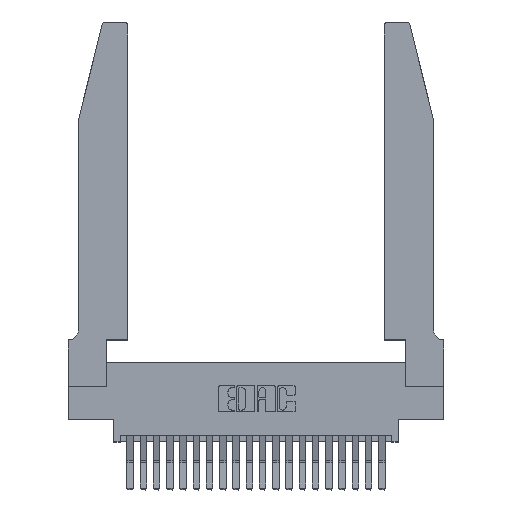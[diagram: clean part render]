
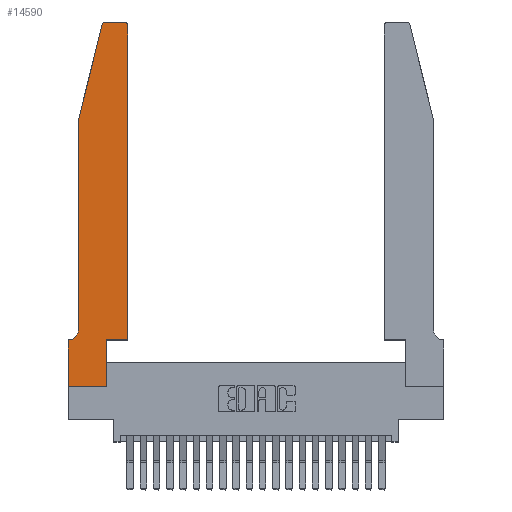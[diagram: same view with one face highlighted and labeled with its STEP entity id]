
A CAD part, top view. The second image highlights one B-rep face of the part: STEP entity #14590.
In plain terms, the highlighted planar face has unit normal (0, 0, 1).
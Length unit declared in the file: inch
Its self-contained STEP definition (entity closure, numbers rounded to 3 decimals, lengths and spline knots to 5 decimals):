
#285 = CARTESIAN_POINT ( 'NONE',  ( 0.4505, 0.35, 0.37 ) ) ;
#601 = VERTEX_POINT ( 'NONE', #14950 ) ;
#890 = LINE ( 'NONE', #285, #14241 ) ;
#1295 = LINE ( 'NONE', #7377, #20092 ) ;
#1777 = CIRCLE ( 'NONE', #19327, 0.03 ) ;
#1810 = VERTEX_POINT ( 'NONE', #23655 ) ;
#1978 = CARTESIAN_POINT ( 'NONE',  ( 0.284, 2.72, 0.37 ) ) ;
#2127 = AXIS2_PLACEMENT_3D ( 'NONE', #1978, #16276, #14726 ) ;
#3044 = LINE ( 'NONE', #10957, #20736 ) ;
#3111 = CARTESIAN_POINT ( 'NONE',  ( 0.0055, 0.35, 0.37 ) ) ;
#3375 = EDGE_CURVE ( 'NONE', #19369, #8964, #22174, .T. ) ;
#3530 = CARTESIAN_POINT ( 'NONE',  ( 0.0755, 2., 0.37 ) ) ;
#3537 = LINE ( 'NONE', #9108, #23262 ) ;
#3721 = LINE ( 'NONE', #5532, #21436 ) ;
#4109 = EDGE_CURVE ( 'NONE', #8964, #20138, #1295, .T. ) ;
#4708 = VECTOR ( 'NONE', #10912, 39.37008 ) ;
#5532 = CARTESIAN_POINT ( 'NONE',  ( 0.0755, 2., 0.37 ) ) ;
#5717 = EDGE_CURVE ( 'NONE', #11698, #6690, #1777, .T. ) ;
#5943 = CARTESIAN_POINT ( 'NONE',  ( 0.2865, 0., 0.37 ) ) ;
#6015 = VERTEX_POINT ( 'NONE', #3111 ) ;
#6218 = DIRECTION ( 'NONE',  ( 0., 0., -1. ) ) ;
#6465 = CARTESIAN_POINT ( 'NONE',  ( 0., 0., 0.37 ) ) ;
#6519 = DIRECTION ( 'NONE',  ( 0., 0., 1. ) ) ;
#6690 = VERTEX_POINT ( 'NONE', #17629 ) ;
#6797 = CARTESIAN_POINT ( 'NONE',  ( 0., 0.35, 0.37 ) ) ;
#6894 = DIRECTION ( 'NONE',  ( 1., 0., 0. ) ) ;
#7010 = VECTOR ( 'NONE', #17086, 39.37008 ) ;
#7377 = CARTESIAN_POINT ( 'NONE',  ( 0., 0., 0.37 ) ) ;
#7633 = ORIENTED_EDGE ( 'NONE', *, *, #7678, .T. ) ;
#7678 = EDGE_CURVE ( 'NONE', #6015, #19369, #12638, .T. ) ;
#7726 = ORIENTED_EDGE ( 'NONE', *, *, #22436, .T. ) ;
#7731 = DIRECTION ( 'NONE',  ( -1., 0., 0. ) ) ;
#8350 = CARTESIAN_POINT ( 'NONE',  ( 0.284, 2.75, 0.37 ) ) ;
#8524 = CARTESIAN_POINT ( 'NONE',  ( 0., 0.35, 0.37 ) ) ;
#8791 = ORIENTED_EDGE ( 'NONE', *, *, #10502, .T. ) ;
#8905 = EDGE_CURVE ( 'NONE', #19988, #6015, #12291, .T. ) ;
#8915 = ORIENTED_EDGE ( 'NONE', *, *, #17233, .T. ) ;
#8924 = ORIENTED_EDGE ( 'NONE', *, *, #3375, .T. ) ;
#8964 = VERTEX_POINT ( 'NONE', #20673 ) ;
#9101 = VECTOR ( 'NONE', #20529, 39.37008 ) ;
#9108 = CARTESIAN_POINT ( 'NONE',  ( 0.2865, 0.35, 0.37 ) ) ;
#10080 = ORIENTED_EDGE ( 'NONE', *, *, #16551, .T. ) ;
#10502 = EDGE_CURVE ( 'NONE', #601, #16322, #22596, .T. ) ;
#10912 = DIRECTION ( 'NONE',  ( 0., -1., 0. ) ) ;
#10957 = CARTESIAN_POINT ( 'NONE',  ( 0.4505, 0.35, 0.37 ) ) ;
#11335 = CARTESIAN_POINT ( 'NONE',  ( 0.0755, 2., 0.37 ) ) ;
#11579 = ORIENTED_EDGE ( 'NONE', *, *, #13323, .T. ) ;
#11635 = DIRECTION ( 'NONE',  ( 0., 0., 1. ) ) ;
#11698 = VERTEX_POINT ( 'NONE', #20139 ) ;
#11709 = DIRECTION ( 'NONE',  ( 0., 1., 0. ) ) ;
#11810 = LINE ( 'NONE', #20707, #7010 ) ;
#12139 = ORIENTED_EDGE ( 'NONE', *, *, #13207, .T. ) ;
#12179 = FACE_OUTER_BOUND ( 'NONE', #15539, .T. ) ;
#12199 = ORIENTED_EDGE ( 'NONE', *, *, #8905, .T. ) ;
#12291 = CIRCLE ( 'NONE', #18557, 0.07 ) ;
#12638 = LINE ( 'NONE', #19195, #16895 ) ;
#12712 = CARTESIAN_POINT ( 'NONE',  ( 0.2865, 0.35, 0.37 ) ) ;
#13207 = EDGE_CURVE ( 'NONE', #16322, #19988, #3721, .T. ) ;
#13323 = EDGE_CURVE ( 'NONE', #16166, #1810, #890, .T. ) ;
#13511 = DIRECTION ( 'NONE',  ( -1., 0., 0. ) ) ;
#13555 = ORIENTED_EDGE ( 'NONE', *, *, #22484, .T. ) ;
#14241 = VECTOR ( 'NONE', #6894, 39.37008 ) ;
#14590 = ADVANCED_FACE ( 'NONE', ( #12179 ), #15591, .T. ) ;
#14607 = ORIENTED_EDGE ( 'NONE', *, *, #4109, .T. ) ;
#14726 = DIRECTION ( 'NONE',  ( 1., 0., 0. ) ) ;
#14950 = CARTESIAN_POINT ( 'NONE',  ( 0.25487, 2.72718, 0.37 ) ) ;
#15539 = EDGE_LOOP ( 'NONE', ( #8915, #13555, #8791, #12139, #12199, #7633, #8924, #14607, #7726, #11579, #10080, #21323 ) ) ;
#15591 = PLANE ( 'NONE',  #19555 ) ;
#16166 = VERTEX_POINT ( 'NONE', #12712 ) ;
#16276 = DIRECTION ( 'NONE',  ( 0., 0., 1. ) ) ;
#16322 = VERTEX_POINT ( 'NONE', #3530 ) ;
#16329 = CIRCLE ( 'NONE', #2127, 0.03 ) ;
#16551 = EDGE_CURVE ( 'NONE', #1810, #11698, #3044, .T. ) ;
#16895 = VECTOR ( 'NONE', #13511, 39.37008 ) ;
#17060 = CARTESIAN_POINT ( 'NONE',  ( 0.4205, 2.72, 0.37 ) ) ;
#17086 = DIRECTION ( 'NONE',  ( -1., 0., 0. ) ) ;
#17233 = EDGE_CURVE ( 'NONE', #6690, #23499, #11810, .T. ) ;
#17629 = CARTESIAN_POINT ( 'NONE',  ( 0.4205, 2.75, 0.37 ) ) ;
#17839 = DIRECTION ( 'NONE',  ( 0., -1., 0. ) ) ;
#18115 = DIRECTION ( 'NONE',  ( 0., 1., 0. ) ) ;
#18557 = AXIS2_PLACEMENT_3D ( 'NONE', #20589, #6218, #7731 ) ;
#18974 = DIRECTION ( 'NONE',  ( 1., 0., 0. ) ) ;
#19195 = CARTESIAN_POINT ( 'NONE',  ( 0.0755, 0.35, 0.37 ) ) ;
#19288 = DIRECTION ( 'NONE',  ( 1., 0., 0. ) ) ;
#19327 = AXIS2_PLACEMENT_3D ( 'NONE', #17060, #11635, #18974 ) ;
#19369 = VERTEX_POINT ( 'NONE', #6797 ) ;
#19555 = AXIS2_PLACEMENT_3D ( 'NONE', #8524, #6519, #19288 ) ;
#19927 = CARTESIAN_POINT ( 'NONE',  ( 0.0755, 0.42, 0.37 ) ) ;
#19988 = VERTEX_POINT ( 'NONE', #19927 ) ;
#20092 = VECTOR ( 'NONE', #20356, 39.37008 ) ;
#20138 = VERTEX_POINT ( 'NONE', #5943 ) ;
#20139 = CARTESIAN_POINT ( 'NONE',  ( 0.4505, 2.72, 0.37 ) ) ;
#20356 = DIRECTION ( 'NONE',  ( 1., 0., 0. ) ) ;
#20529 = DIRECTION ( 'NONE',  ( -0.239, -0.971, 0. ) ) ;
#20589 = CARTESIAN_POINT ( 'NONE',  ( 0.0055, 0.42, 0.37 ) ) ;
#20673 = CARTESIAN_POINT ( 'NONE',  ( 0., 0., 0.37 ) ) ;
#20707 = CARTESIAN_POINT ( 'NONE',  ( 0.2605, 2.75, 0.37 ) ) ;
#20736 = VECTOR ( 'NONE', #11709, 39.37008 ) ;
#21323 = ORIENTED_EDGE ( 'NONE', *, *, #5717, .T. ) ;
#21436 = VECTOR ( 'NONE', #17839, 39.37008 ) ;
#22174 = LINE ( 'NONE', #6465, #4708 ) ;
#22436 = EDGE_CURVE ( 'NONE', #20138, #16166, #3537, .T. ) ;
#22484 = EDGE_CURVE ( 'NONE', #23499, #601, #16329, .T. ) ;
#22596 = LINE ( 'NONE', #11335, #9101 ) ;
#23262 = VECTOR ( 'NONE', #18115, 39.37008 ) ;
#23499 = VERTEX_POINT ( 'NONE', #8350 ) ;
#23655 = CARTESIAN_POINT ( 'NONE',  ( 0.4505, 0.35, 0.37 ) ) ;
